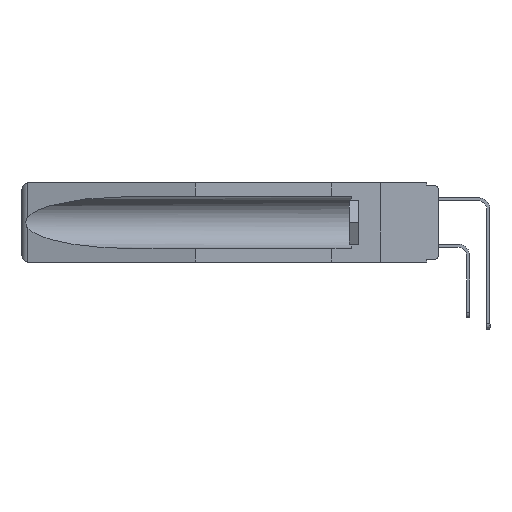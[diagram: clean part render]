
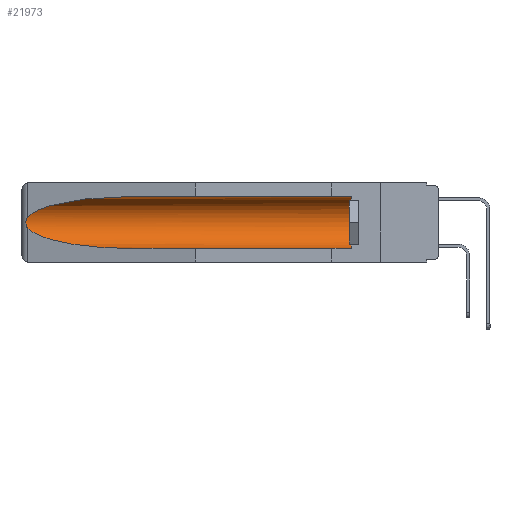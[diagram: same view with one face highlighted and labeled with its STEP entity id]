
A CAD part, left-side view. The second image highlights one B-rep face of the part: STEP entity #21973.
In plain terms, the highlighted cylindrical face has radius 2.857 mm (diameter 5.715 mm), a partial arc.
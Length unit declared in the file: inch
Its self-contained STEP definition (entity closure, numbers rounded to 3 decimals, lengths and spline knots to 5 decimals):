
#22 = CARTESIAN_POINT ( 'NONE',  ( 0.155, 0.126, -0.059 ) ) ;
#493 = ORIENTED_EDGE ( 'NONE', *, *, #14096, .F. ) ;
#1207 = VERTEX_POINT ( 'NONE', #13616 ) ;
#1214 = CARTESIAN_POINT ( 'NONE',  ( 0.155, 0.126, -0.284 ) ) ;
#1525 =( BOUNDED_CURVE ( )  B_SPLINE_CURVE ( 3, ( #2371, #14736, #7785, #9629 ),
 .UNSPECIFIED., .F., .T. ) 
 B_SPLINE_CURVE_WITH_KNOTS ( ( 4, 4 ),
 ( 0.1948, 1.5708 ),
 .UNSPECIFIED. ) 
 CURVE ( )  GEOMETRIC_REPRESENTATION_ITEM ( )  RATIONAL_B_SPLINE_CURVE ( ( 1., 0.848, 0.848, 1. ) ) 
 REPRESENTATION_ITEM ( '' )  );
#2227 = CARTESIAN_POINT ( 'NONE',  ( 0.155, -0.30754, -0.059 ) ) ;
#2371 = CARTESIAN_POINT ( 'NONE',  ( 0.26537, 1.52718, -0.19328 ) ) ;
#2893 = CIRCLE ( 'NONE', #14707, 0.1125 ) ;
#4060 = CARTESIAN_POINT ( 'NONE',  ( 0.155, 0.126, -0.1715 ) ) ;
#4332 = CARTESIAN_POINT ( 'NONE',  ( 0.2675, 1.53308, -0.17534 ) ) ;
#4408 = ORIENTED_EDGE ( 'NONE', *, *, #11952, .T. ) ;
#4534 = CARTESIAN_POINT ( 'NONE',  ( 0.25451, 1.48313, -0.09465 ) ) ;
#5091 = VECTOR ( 'NONE', #21312, 39.37008 ) ;
#5565 = LINE ( 'NONE', #19686, #16123 ) ;
#6009 = EDGE_CURVE ( 'NONE', #17893, #20300, #2893, .T. ) ;
#6083 = CARTESIAN_POINT ( 'NONE',  ( 0.26597, 1.5296, -0.19026 ) ) ;
#6478 = ORIENTED_EDGE ( 'NONE', *, *, #6009, .T. ) ;
#7785 = CARTESIAN_POINT ( 'NONE',  ( 0.21114, 1.30732, -0.284 ) ) ;
#8289 = CARTESIAN_POINT ( 'NONE',  ( 0.155, 1.07973, -0.059 ) ) ;
#8885 = FACE_OUTER_BOUND ( 'NONE', #16913, .T. ) ;
#9315 = CARTESIAN_POINT ( 'NONE',  ( 0.26597, 1.52961, -0.15275 ) ) ;
#9375 = DIRECTION ( 'NONE',  ( 0., -1., 0. ) ) ;
#9506 = CARTESIAN_POINT ( 'NONE',  ( 0.26537, 1.52718, -0.14972 ) ) ;
#9629 = CARTESIAN_POINT ( 'NONE',  ( 0.155, 1.07973, -0.284 ) ) ;
#10404 = DIRECTION ( 'NONE',  ( 0., 1., 0. ) ) ;
#10533 = VERTEX_POINT ( 'NONE', #21320 ) ;
#11393 = CARTESIAN_POINT ( 'NONE',  ( 0.26537, 1.52718, -0.19328 ) ) ;
#11952 = EDGE_CURVE ( 'NONE', #18628, #10533, #17304, .T. ) ;
#12263 = ORIENTED_EDGE ( 'NONE', *, *, #20187, .T. ) ;
#12645 = LINE ( 'NONE', #2227, #5091 ) ;
#12915 = CARTESIAN_POINT ( 'NONE',  ( 0.26655, 1.53094, -0.18657 ) ) ;
#13177 = EDGE_CURVE ( 'NONE', #10533, #19814, #13526, .T. ) ;
#13323 = CARTESIAN_POINT ( 'NONE',  ( 0.21114, 1.30732, -0.059 ) ) ;
#13526 = B_SPLINE_CURVE_WITH_KNOTS ( 'NONE', 3,
 ( #19962, #9315, #14861, #17978, #19737, #4332, #21940, #12915, #6083, #11393 ),
 .UNSPECIFIED., .F., .F.,
 ( 4, 2, 2, 2, 4 ),
 ( 0., 0.00029, 0.00058, 0.00087, 0.00117 ),
 .UNSPECIFIED. ) ;
#13616 = CARTESIAN_POINT ( 'NONE',  ( 0.155, 1.07973, -0.284 ) ) ;
#13772 = ORIENTED_EDGE ( 'NONE', *, *, #19886, .T. ) ;
#14096 = EDGE_CURVE ( 'NONE', #17893, #1207, #5565, .T. ) ;
#14216 = CYLINDRICAL_SURFACE ( 'NONE', #18395, 0.1125 ) ;
#14451 = CARTESIAN_POINT ( 'NONE',  ( 0.155, -0.30754, -0.1715 ) ) ;
#14707 = AXIS2_PLACEMENT_3D ( 'NONE', #4060, #9375, #16426 ) ;
#14736 = CARTESIAN_POINT ( 'NONE',  ( 0.25451, 1.48313, -0.24835 ) ) ;
#14861 = CARTESIAN_POINT ( 'NONE',  ( 0.26654, 1.53092, -0.15636 ) ) ;
#14937 = CARTESIAN_POINT ( 'NONE',  ( 0.155, 1.07973, -0.059 ) ) ;
#16123 = VECTOR ( 'NONE', #10404, 39.37008 ) ;
#16426 = DIRECTION ( 'NONE',  ( 0., 0., 1. ) ) ;
#16913 = EDGE_LOOP ( 'NONE', ( #4408, #17791, #13772, #493, #6478, #12263 ) ) ;
#17304 =( BOUNDED_CURVE ( )  B_SPLINE_CURVE ( 3, ( #14937, #13323, #4534, #9506 ),
 .UNSPECIFIED., .F., .T. ) 
 B_SPLINE_CURVE_WITH_KNOTS ( ( 4, 4 ),
 ( 4.71239, 6.08839 ),
 .UNSPECIFIED. ) 
 CURVE ( )  GEOMETRIC_REPRESENTATION_ITEM ( )  RATIONAL_B_SPLINE_CURVE ( ( 1., 0.848, 0.848, 1. ) ) 
 REPRESENTATION_ITEM ( '' )  );
#17791 = ORIENTED_EDGE ( 'NONE', *, *, #13177, .T. ) ;
#17893 = VERTEX_POINT ( 'NONE', #1214 ) ;
#17978 = CARTESIAN_POINT ( 'NONE',  ( 0.2673, 1.5327, -0.16383 ) ) ;
#18145 = DIRECTION ( 'NONE',  ( 0., 1., 0. ) ) ;
#18395 = AXIS2_PLACEMENT_3D ( 'NONE', #14451, #18145, #21284 ) ;
#18628 = VERTEX_POINT ( 'NONE', #8289 ) ;
#19608 = CARTESIAN_POINT ( 'NONE',  ( 0.26537, 1.52718, -0.19328 ) ) ;
#19686 = CARTESIAN_POINT ( 'NONE',  ( 0.155, -0.30754, -0.284 ) ) ;
#19737 = CARTESIAN_POINT ( 'NONE',  ( 0.2675, 1.53308, -0.16763 ) ) ;
#19814 = VERTEX_POINT ( 'NONE', #19608 ) ;
#19886 = EDGE_CURVE ( 'NONE', #19814, #1207, #1525, .T. ) ;
#19962 = CARTESIAN_POINT ( 'NONE',  ( 0.26537, 1.52718, -0.14972 ) ) ;
#20187 = EDGE_CURVE ( 'NONE', #20300, #18628, #12645, .T. ) ;
#20300 = VERTEX_POINT ( 'NONE', #22 ) ;
#21284 = DIRECTION ( 'NONE',  ( 0., 0., 1. ) ) ;
#21312 = DIRECTION ( 'NONE',  ( 0., 1., 0. ) ) ;
#21320 = CARTESIAN_POINT ( 'NONE',  ( 0.26537, 1.52718, -0.14972 ) ) ;
#21940 = CARTESIAN_POINT ( 'NONE',  ( 0.2673, 1.53269, -0.17917 ) ) ;
#21973 = ADVANCED_FACE ( 'NONE', ( #8885 ), #14216, .F. ) ;
